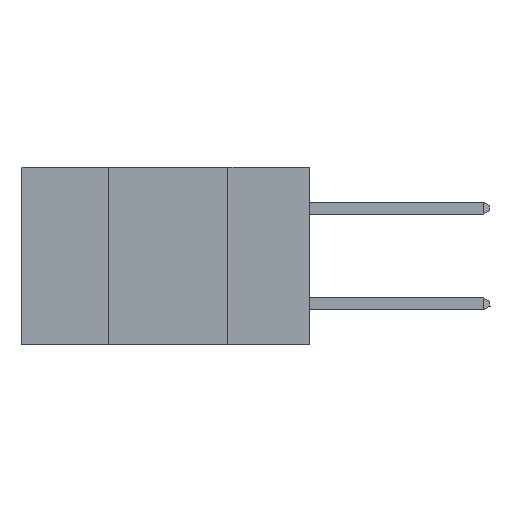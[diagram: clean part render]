
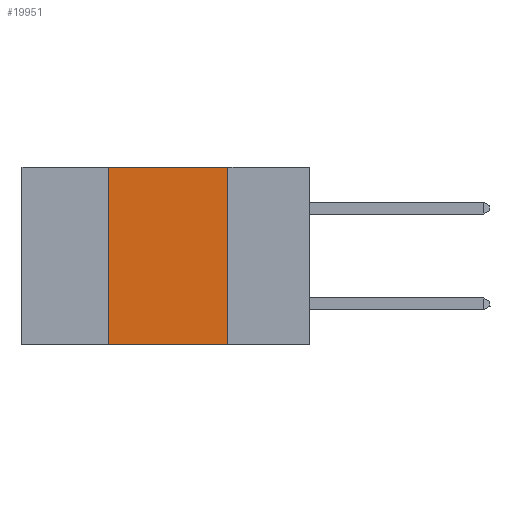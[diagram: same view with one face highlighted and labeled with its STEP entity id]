
A CAD part, left-side view. The second image highlights one B-rep face of the part: STEP entity #19951.
In plain terms, the highlighted planar face has unit normal (-1, 0, 0).
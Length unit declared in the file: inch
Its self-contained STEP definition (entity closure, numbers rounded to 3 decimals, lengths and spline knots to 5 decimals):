
#749 = VERTEX_POINT ( 'NONE', #17579 ) ;
#1459 = EDGE_CURVE ( 'NONE', #23075, #20659, #13579, .T. ) ;
#1699 = DIRECTION ( 'NONE',  ( 0., 0., -1. ) ) ;
#2316 = CARTESIAN_POINT ( 'NONE',  ( 0., 0.17, 0. ) ) ;
#2397 = ORIENTED_EDGE ( 'NONE', *, *, #18782, .F. ) ;
#5992 = CARTESIAN_POINT ( 'NONE',  ( 0., 0.42, 0. ) ) ;
#6315 = CARTESIAN_POINT ( 'NONE',  ( 0., 0.17, 0. ) ) ;
#8483 = DIRECTION ( 'NONE',  ( 0., 0., 1. ) ) ;
#8542 = DIRECTION ( 'NONE',  ( 0., -1., 0. ) ) ;
#10942 = ORIENTED_EDGE ( 'NONE', *, *, #1459, .F. ) ;
#11944 = EDGE_CURVE ( 'NONE', #14956, #749, #26443, .T. ) ;
#12624 = ORIENTED_EDGE ( 'NONE', *, *, #15989, .F. ) ;
#12863 = LINE ( 'NONE', #5992, #25305 ) ;
#13386 = EDGE_LOOP ( 'NONE', ( #2397, #10942, #12624, #20035 ) ) ;
#13579 = LINE ( 'NONE', #14116, #24878 ) ;
#14116 = CARTESIAN_POINT ( 'NONE',  ( 0., 0.6, 0. ) ) ;
#14503 = PLANE ( 'NONE',  #20120 ) ;
#14733 = LINE ( 'NONE', #6315, #31477 ) ;
#14734 = CARTESIAN_POINT ( 'NONE',  ( 0., 0.6, 0. ) ) ;
#14913 = VECTOR ( 'NONE', #21791, 39.37008 ) ;
#14956 = VERTEX_POINT ( 'NONE', #26961 ) ;
#15989 = EDGE_CURVE ( 'NONE', #14956, #23075, #12863, .T. ) ;
#17579 = CARTESIAN_POINT ( 'NONE',  ( 0., 0.17, -0.37 ) ) ;
#18537 = FACE_OUTER_BOUND ( 'NONE', #13386, .T. ) ;
#18782 = EDGE_CURVE ( 'NONE', #20659, #749, #14733, .T. ) ;
#19951 = ADVANCED_FACE ( 'NONE', ( #18537 ), #14503, .F. ) ;
#20035 = ORIENTED_EDGE ( 'NONE', *, *, #11944, .T. ) ;
#20120 = AXIS2_PLACEMENT_3D ( 'NONE', #14734, #24478, #25255 ) ;
#20290 = CARTESIAN_POINT ( 'NONE',  ( 0., 0.42, 0. ) ) ;
#20659 = VERTEX_POINT ( 'NONE', #2316 ) ;
#21791 = DIRECTION ( 'NONE',  ( 0., -1., 0. ) ) ;
#23075 = VERTEX_POINT ( 'NONE', #20290 ) ;
#24423 = CARTESIAN_POINT ( 'NONE',  ( 0., 0.6, -0.37 ) ) ;
#24478 = DIRECTION ( 'NONE',  ( 1., 0., 0. ) ) ;
#24878 = VECTOR ( 'NONE', #8542, 39.37008 ) ;
#25255 = DIRECTION ( 'NONE',  ( 0., 0., -1. ) ) ;
#25305 = VECTOR ( 'NONE', #8483, 39.37008 ) ;
#26443 = LINE ( 'NONE', #24423, #14913 ) ;
#26961 = CARTESIAN_POINT ( 'NONE',  ( 0., 0.42, -0.37 ) ) ;
#31477 = VECTOR ( 'NONE', #1699, 39.37008 ) ;
